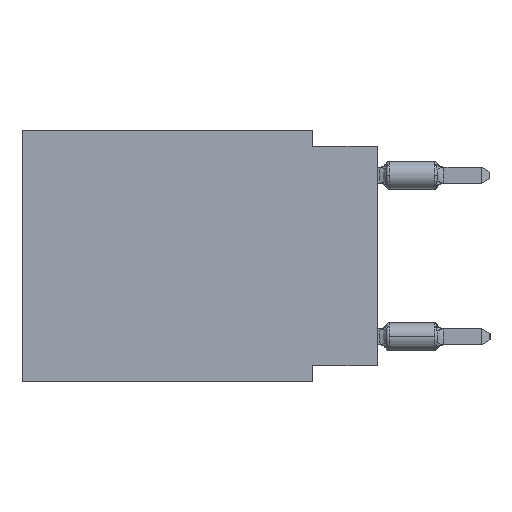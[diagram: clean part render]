
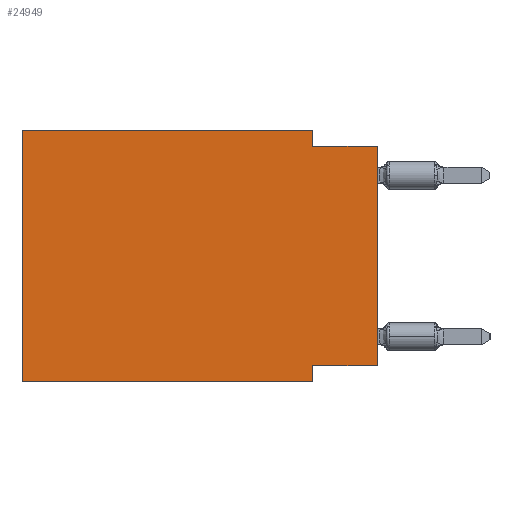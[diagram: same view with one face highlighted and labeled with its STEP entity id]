
A CAD part, left-side view. The second image highlights one B-rep face of the part: STEP entity #24949.
In plain terms, the highlighted planar face has unit normal (-1, 0, 0).
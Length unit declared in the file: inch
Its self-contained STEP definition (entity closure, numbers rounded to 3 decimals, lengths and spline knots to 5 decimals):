
#235 = CARTESIAN_POINT ( 'NONE',  ( 0., 0., 0. ) ) ;
#664 = LINE ( 'NONE', #33897, #3001 ) ;
#1156 = EDGE_LOOP ( 'NONE', ( #25854, #1907, #26734, #1644, #15812, #33621, #11075, #13511 ) ) ;
#1433 = LINE ( 'NONE', #11399, #21421 ) ;
#1644 = ORIENTED_EDGE ( 'NONE', *, *, #14091, .F. ) ;
#1907 = ORIENTED_EDGE ( 'NONE', *, *, #27822, .F. ) ;
#2144 = DIRECTION ( 'NONE',  ( 0., -1., 0. ) ) ;
#2381 = CARTESIAN_POINT ( 'NONE',  ( 0., 0., -0.365 ) ) ;
#2878 = VERTEX_POINT ( 'NONE', #24543 ) ;
#3001 = VECTOR ( 'NONE', #11140, 39.37008 ) ;
#3079 = VECTOR ( 'NONE', #32064, 39.37008 ) ;
#4141 = VECTOR ( 'NONE', #10717, 39.37008 ) ;
#6899 = EDGE_CURVE ( 'NONE', #34002, #8206, #31667, .T. ) ;
#7521 = VECTOR ( 'NONE', #19113, 39.37008 ) ;
#7537 = DIRECTION ( 'NONE',  ( 1., 0., 0. ) ) ;
#8206 = VERTEX_POINT ( 'NONE', #11876 ) ;
#8903 = CARTESIAN_POINT ( 'NONE',  ( 0., 0.1, -0.39 ) ) ;
#9641 = VERTEX_POINT ( 'NONE', #23551 ) ;
#10284 = EDGE_CURVE ( 'NONE', #2878, #22917, #27827, .T. ) ;
#10717 = DIRECTION ( 'NONE',  ( 0., 0., 1. ) ) ;
#11075 = ORIENTED_EDGE ( 'NONE', *, *, #10284, .F. ) ;
#11140 = DIRECTION ( 'NONE',  ( 0., 1., 0. ) ) ;
#11399 = CARTESIAN_POINT ( 'NONE',  ( 0., 0.55, 0. ) ) ;
#11876 = CARTESIAN_POINT ( 'NONE',  ( 0., 0.55, 0. ) ) ;
#11936 = VERTEX_POINT ( 'NONE', #27955 ) ;
#13511 = ORIENTED_EDGE ( 'NONE', *, *, #28444, .F. ) ;
#13855 = VERTEX_POINT ( 'NONE', #2381 ) ;
#14091 = EDGE_CURVE ( 'NONE', #8206, #11936, #1433, .T. ) ;
#14276 = CARTESIAN_POINT ( 'NONE',  ( 0., 0.55, -0.39 ) ) ;
#15360 = CARTESIAN_POINT ( 'NONE',  ( 0., 0.1, -0.39 ) ) ;
#15735 = LINE ( 'NONE', #29298, #33438 ) ;
#15812 = ORIENTED_EDGE ( 'NONE', *, *, #6899, .F. ) ;
#17349 = DIRECTION ( 'NONE',  ( 0., 0., -1. ) ) ;
#17437 = LINE ( 'NONE', #25331, #18306 ) ;
#18306 = VECTOR ( 'NONE', #2144, 39.37008 ) ;
#19113 = DIRECTION ( 'NONE',  ( 0., 0., 1. ) ) ;
#19377 = DIRECTION ( 'NONE',  ( 0., 0., -1. ) ) ;
#20137 = EDGE_CURVE ( 'NONE', #34002, #22917, #15735, .T. ) ;
#20269 = CARTESIAN_POINT ( 'NONE',  ( 0., 0.55, 0. ) ) ;
#21421 = VECTOR ( 'NONE', #29791, 39.37008 ) ;
#22917 = VERTEX_POINT ( 'NONE', #15360 ) ;
#23551 = CARTESIAN_POINT ( 'NONE',  ( 0., 0., -0.025 ) ) ;
#23933 = CARTESIAN_POINT ( 'NONE',  ( 0., 0.55, 0. ) ) ;
#24543 = CARTESIAN_POINT ( 'NONE',  ( 0., 0.1, -0.365 ) ) ;
#24949 = ADVANCED_FACE ( 'NONE', ( #31267 ), #25602, .F. ) ;
#25331 = CARTESIAN_POINT ( 'NONE',  ( 0., 0., -0.025 ) ) ;
#25602 = PLANE ( 'NONE',  #31914 ) ;
#25854 = ORIENTED_EDGE ( 'NONE', *, *, #29313, .T. ) ;
#26196 = LINE ( 'NONE', #235, #4141 ) ;
#26206 = VERTEX_POINT ( 'NONE', #30357 ) ;
#26378 = DIRECTION ( 'NONE',  ( 0., -1., 0. ) ) ;
#26734 = ORIENTED_EDGE ( 'NONE', *, *, #31239, .F. ) ;
#27822 = EDGE_CURVE ( 'NONE', #26206, #9641, #17437, .T. ) ;
#27827 = LINE ( 'NONE', #8903, #27984 ) ;
#27955 = CARTESIAN_POINT ( 'NONE',  ( 0., 0.1, 0. ) ) ;
#27984 = VECTOR ( 'NONE', #17349, 39.37008 ) ;
#28444 = EDGE_CURVE ( 'NONE', #13855, #2878, #664, .T. ) ;
#29123 = CARTESIAN_POINT ( 'NONE',  ( 0., 0.1, 0. ) ) ;
#29298 = CARTESIAN_POINT ( 'NONE',  ( 0., 0.55, -0.39 ) ) ;
#29313 = EDGE_CURVE ( 'NONE', #13855, #9641, #26196, .T. ) ;
#29641 = LINE ( 'NONE', #29123, #3079 ) ;
#29791 = DIRECTION ( 'NONE',  ( 0., -1., 0. ) ) ;
#30357 = CARTESIAN_POINT ( 'NONE',  ( 0., 0.1, -0.025 ) ) ;
#31239 = EDGE_CURVE ( 'NONE', #11936, #26206, #29641, .T. ) ;
#31267 = FACE_OUTER_BOUND ( 'NONE', #1156, .T. ) ;
#31667 = LINE ( 'NONE', #23933, #7521 ) ;
#31914 = AXIS2_PLACEMENT_3D ( 'NONE', #20269, #7537, #19377 ) ;
#32064 = DIRECTION ( 'NONE',  ( 0., 0., -1. ) ) ;
#33438 = VECTOR ( 'NONE', #26378, 39.37008 ) ;
#33621 = ORIENTED_EDGE ( 'NONE', *, *, #20137, .T. ) ;
#33897 = CARTESIAN_POINT ( 'NONE',  ( 0., 0., -0.365 ) ) ;
#34002 = VERTEX_POINT ( 'NONE', #14276 ) ;
